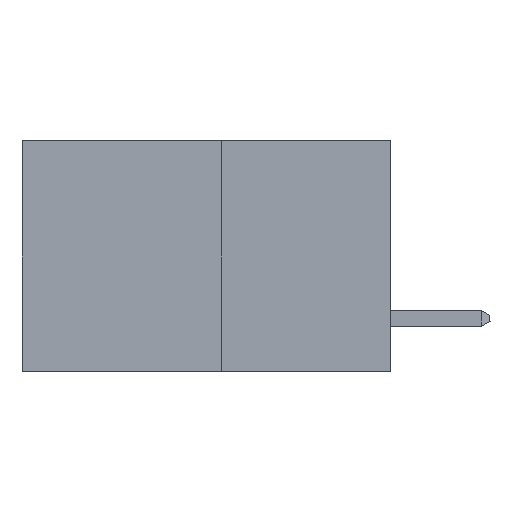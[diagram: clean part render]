
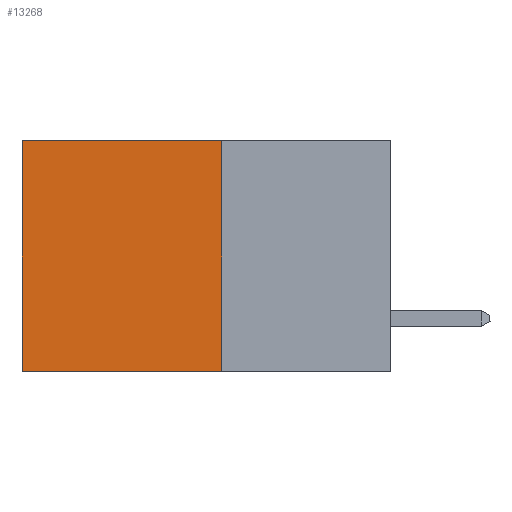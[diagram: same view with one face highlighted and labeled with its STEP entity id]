
A CAD part, left-side view. The second image highlights one B-rep face of the part: STEP entity #13268.
In plain terms, the highlighted planar face has unit normal (-1, 0, 0).
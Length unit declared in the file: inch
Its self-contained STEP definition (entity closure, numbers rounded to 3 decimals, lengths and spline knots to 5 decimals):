
#459 = CARTESIAN_POINT ( 'NONE',  ( 0.277, 0.59, -0.37 ) ) ;
#1004 = VERTEX_POINT ( 'NONE', #13795 ) ;
#1070 = DIRECTION ( 'NONE',  ( 0., 1., 0. ) ) ;
#1071 = DIRECTION ( 'NONE',  ( 0., 0., -1. ) ) ;
#1083 = VERTEX_POINT ( 'NONE', #9861 ) ;
#1151 = FACE_OUTER_BOUND ( 'NONE', #7302, .T. ) ;
#1306 = LINE ( 'NONE', #459, #6511 ) ;
#1438 = CARTESIAN_POINT ( 'NONE',  ( 0.277, 0.27, -0.37 ) ) ;
#2370 = ORIENTED_EDGE ( 'NONE', *, *, #10935, .T. ) ;
#2697 = EDGE_CURVE ( 'NONE', #1083, #12767, #12639, .T. ) ;
#2761 = ORIENTED_EDGE ( 'NONE', *, *, #12895, .T. ) ;
#2825 = DIRECTION ( 'NONE',  ( 0., 0., -1. ) ) ;
#4168 = VECTOR ( 'NONE', #2825, 39.37008 ) ;
#5052 = LINE ( 'NONE', #1438, #10114 ) ;
#5295 = ORIENTED_EDGE ( 'NONE', *, *, #6159, .F. ) ;
#5760 = CARTESIAN_POINT ( 'NONE',  ( 0.277, 0.27, -0.37 ) ) ;
#6159 = EDGE_CURVE ( 'NONE', #12767, #1004, #5052, .T. ) ;
#6383 = CARTESIAN_POINT ( 'NONE',  ( 0.277, 0.59, 0. ) ) ;
#6511 = VECTOR ( 'NONE', #7118, 39.37008 ) ;
#6597 = AXIS2_PLACEMENT_3D ( 'NONE', #13959, #7684, #1071 ) ;
#6617 = PLANE ( 'NONE',  #6597 ) ;
#7118 = DIRECTION ( 'NONE',  ( 0., 0., -1. ) ) ;
#7177 = CARTESIAN_POINT ( 'NONE',  ( 0.277, 0.27, -0.37 ) ) ;
#7188 = CARTESIAN_POINT ( 'NONE',  ( 0.277, 0.27, 0. ) ) ;
#7302 = EDGE_LOOP ( 'NONE', ( #2370, #5295, #8198, #2761 ) ) ;
#7684 = DIRECTION ( 'NONE',  ( 1., 0., 0. ) ) ;
#7846 = VECTOR ( 'NONE', #9325, 39.37008 ) ;
#8198 = ORIENTED_EDGE ( 'NONE', *, *, #2697, .F. ) ;
#8199 = LINE ( 'NONE', #7188, #7846 ) ;
#8864 = VERTEX_POINT ( 'NONE', #6383 ) ;
#9325 = DIRECTION ( 'NONE',  ( 0., 1., 0. ) ) ;
#9861 = CARTESIAN_POINT ( 'NONE',  ( 0.277, 0.27, 0. ) ) ;
#10114 = VECTOR ( 'NONE', #1070, 39.37008 ) ;
#10935 = EDGE_CURVE ( 'NONE', #8864, #1004, #1306, .T. ) ;
#12639 = LINE ( 'NONE', #7177, #4168 ) ;
#12767 = VERTEX_POINT ( 'NONE', #5760 ) ;
#12895 = EDGE_CURVE ( 'NONE', #1083, #8864, #8199, .T. ) ;
#13268 = ADVANCED_FACE ( 'NONE', ( #1151 ), #6617, .F. ) ;
#13795 = CARTESIAN_POINT ( 'NONE',  ( 0.277, 0.59, -0.37 ) ) ;
#13959 = CARTESIAN_POINT ( 'NONE',  ( 0.277, 0.27, -0.37 ) ) ;
